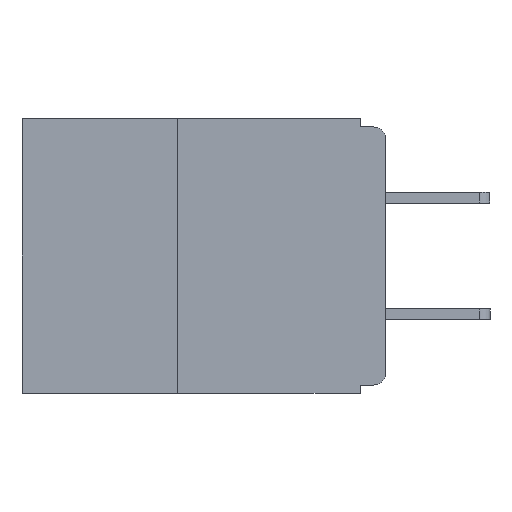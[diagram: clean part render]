
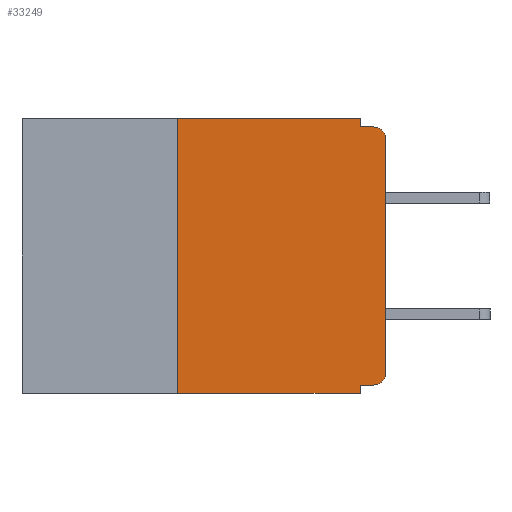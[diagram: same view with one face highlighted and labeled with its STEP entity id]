
A CAD part, left-side view. The second image highlights one B-rep face of the part: STEP entity #33249.
In plain terms, the highlighted planar face has unit normal (-1, 0, 0).
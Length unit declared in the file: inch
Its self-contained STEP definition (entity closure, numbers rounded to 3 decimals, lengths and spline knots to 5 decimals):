
#244 = LINE ( 'NONE', #11708, #6750 ) ;
#290 = ORIENTED_EDGE ( 'NONE', *, *, #3666, .F. ) ;
#354 = VECTOR ( 'NONE', #29643, 39.37008 ) ;
#355 = DIRECTION ( 'NONE',  ( 0., 1., 0. ) ) ;
#597 = CARTESIAN_POINT ( 'NONE',  ( 0., 0.031, -0.33 ) ) ;
#1960 = VERTEX_POINT ( 'NONE', #28369 ) ;
#2477 = AXIS2_PLACEMENT_3D ( 'NONE', #29613, #13690, #32219 ) ;
#2681 = PLANE ( 'NONE',  #2477 ) ;
#2716 = ORIENTED_EDGE ( 'NONE', *, *, #25266, .F. ) ;
#3018 = CIRCLE ( 'NONE', #10564, 0.015 ) ;
#3390 = CARTESIAN_POINT ( 'NONE',  ( 0., 0.031, -0.33 ) ) ;
#3473 = VERTEX_POINT ( 'NONE', #5521 ) ;
#3666 = EDGE_CURVE ( 'NONE', #20793, #1960, #244, .T. ) ;
#4185 = EDGE_CURVE ( 'NONE', #3473, #7208, #5851, .T. ) ;
#5353 = VERTEX_POINT ( 'NONE', #8039 ) ;
#5369 = CARTESIAN_POINT ( 'NONE',  ( 0., 0.015, -0.025 ) ) ;
#5521 = CARTESIAN_POINT ( 'NONE',  ( 0., 0.015, -0.32 ) ) ;
#5851 = LINE ( 'NONE', #16728, #33423 ) ;
#6030 = VECTOR ( 'NONE', #32942, 39.37008 ) ;
#6411 = EDGE_LOOP ( 'NONE', ( #31532, #8694, #2716, #19038, #28151, #290, #25960, #9098, #23011, #10300 ) ) ;
#6750 = VECTOR ( 'NONE', #32842, 39.37008 ) ;
#7208 = VERTEX_POINT ( 'NONE', #25109 ) ;
#7227 = VECTOR ( 'NONE', #34407, 39.37008 ) ;
#7732 = LINE ( 'NONE', #8238, #354 ) ;
#8039 = CARTESIAN_POINT ( 'NONE',  ( 0., 0.031, 0. ) ) ;
#8129 = DIRECTION ( 'NONE',  ( 0., 0., -1. ) ) ;
#8238 = CARTESIAN_POINT ( 'NONE',  ( 0., 0., -0.01 ) ) ;
#8694 = ORIENTED_EDGE ( 'NONE', *, *, #25219, .T. ) ;
#9098 = ORIENTED_EDGE ( 'NONE', *, *, #21715, .F. ) ;
#9358 = VECTOR ( 'NONE', #22515, 39.37008 ) ;
#10300 = ORIENTED_EDGE ( 'NONE', *, *, #30297, .T. ) ;
#10558 = LINE ( 'NONE', #597, #11411 ) ;
#10564 = AXIS2_PLACEMENT_3D ( 'NONE', #5369, #24220, #8129 ) ;
#11127 = VERTEX_POINT ( 'NONE', #3390 ) ;
#11411 = VECTOR ( 'NONE', #16951, 39.37008 ) ;
#11708 = CARTESIAN_POINT ( 'NONE',  ( 0., 0.25, -0.33 ) ) ;
#13141 = CARTESIAN_POINT ( 'NONE',  ( 0., 0.015, -0.305 ) ) ;
#13182 = VERTEX_POINT ( 'NONE', #14042 ) ;
#13690 = DIRECTION ( 'NONE',  ( 1., 0., 0. ) ) ;
#14042 = CARTESIAN_POINT ( 'NONE',  ( 0., 0., -0.025 ) ) ;
#14440 = CIRCLE ( 'NONE', #27930, 0.015 ) ;
#14548 = CARTESIAN_POINT ( 'NONE',  ( 0., 0.437, -0.33 ) ) ;
#15721 = CARTESIAN_POINT ( 'NONE',  ( 0., 0.25, -0.33 ) ) ;
#15816 = DIRECTION ( 'NONE',  ( 0., 0., -1. ) ) ;
#15925 = CARTESIAN_POINT ( 'NONE',  ( 0., 0., 0. ) ) ;
#16463 = CARTESIAN_POINT ( 'NONE',  ( 0., 0.031, -0.01 ) ) ;
#16728 = CARTESIAN_POINT ( 'NONE',  ( 0., 0., -0.32 ) ) ;
#16951 = DIRECTION ( 'NONE',  ( 0., 0., -1. ) ) ;
#17367 = LINE ( 'NONE', #14548, #9358 ) ;
#17755 = VERTEX_POINT ( 'NONE', #16463 ) ;
#19038 = ORIENTED_EDGE ( 'NONE', *, *, #24900, .F. ) ;
#19845 = LINE ( 'NONE', #15925, #7227 ) ;
#20793 = VERTEX_POINT ( 'NONE', #15721 ) ;
#21715 = EDGE_CURVE ( 'NONE', #7208, #11127, #10558, .T. ) ;
#22391 = FACE_OUTER_BOUND ( 'NONE', #6411, .T. ) ;
#22515 = DIRECTION ( 'NONE',  ( 0., -1., 0. ) ) ;
#23011 = ORIENTED_EDGE ( 'NONE', *, *, #4185, .F. ) ;
#23873 = DIRECTION ( 'NONE',  ( 0., -1., 0. ) ) ;
#24220 = DIRECTION ( 'NONE',  ( -1., 0., 0. ) ) ;
#24900 = EDGE_CURVE ( 'NONE', #5353, #17755, #27489, .T. ) ;
#24905 = CARTESIAN_POINT ( 'NONE',  ( 0., 0.015, -0.01 ) ) ;
#25109 = CARTESIAN_POINT ( 'NONE',  ( 0., 0.031, -0.32 ) ) ;
#25146 = EDGE_CURVE ( 'NONE', #1960, #5353, #33176, .T. ) ;
#25219 = EDGE_CURVE ( 'NONE', #13182, #32692, #3018, .T. ) ;
#25266 = EDGE_CURVE ( 'NONE', #17755, #32692, #7732, .T. ) ;
#25960 = ORIENTED_EDGE ( 'NONE', *, *, #30003, .T. ) ;
#26224 = VECTOR ( 'NONE', #23873, 39.37008 ) ;
#27489 = LINE ( 'NONE', #30334, #6030 ) ;
#27610 = CARTESIAN_POINT ( 'NONE',  ( 0., 0., -0.305 ) ) ;
#27930 = AXIS2_PLACEMENT_3D ( 'NONE', #13141, #31689, #15816 ) ;
#28151 = ORIENTED_EDGE ( 'NONE', *, *, #25146, .F. ) ;
#28369 = CARTESIAN_POINT ( 'NONE',  ( 0., 0.25, 0. ) ) ;
#28602 = CARTESIAN_POINT ( 'NONE',  ( 0., 0.437, 0. ) ) ;
#29613 = CARTESIAN_POINT ( 'NONE',  ( 0., 0.437, 0. ) ) ;
#29643 = DIRECTION ( 'NONE',  ( 0., -1., 0. ) ) ;
#30003 = EDGE_CURVE ( 'NONE', #20793, #11127, #17367, .T. ) ;
#30297 = EDGE_CURVE ( 'NONE', #3473, #32196, #14440, .T. ) ;
#30334 = CARTESIAN_POINT ( 'NONE',  ( 0., 0.031, 0. ) ) ;
#30340 = EDGE_CURVE ( 'NONE', #32196, #13182, #19845, .T. ) ;
#31532 = ORIENTED_EDGE ( 'NONE', *, *, #30340, .T. ) ;
#31689 = DIRECTION ( 'NONE',  ( -1., 0., 0. ) ) ;
#32196 = VERTEX_POINT ( 'NONE', #27610 ) ;
#32219 = DIRECTION ( 'NONE',  ( 0., 0., -1. ) ) ;
#32692 = VERTEX_POINT ( 'NONE', #24905 ) ;
#32842 = DIRECTION ( 'NONE',  ( 0., 0., 1. ) ) ;
#32942 = DIRECTION ( 'NONE',  ( 0., 0., -1. ) ) ;
#33176 = LINE ( 'NONE', #28602, #26224 ) ;
#33249 = ADVANCED_FACE ( 'NONE', ( #22391 ), #2681, .F. ) ;
#33423 = VECTOR ( 'NONE', #355, 39.37008 ) ;
#34407 = DIRECTION ( 'NONE',  ( 0., 0., 1. ) ) ;
